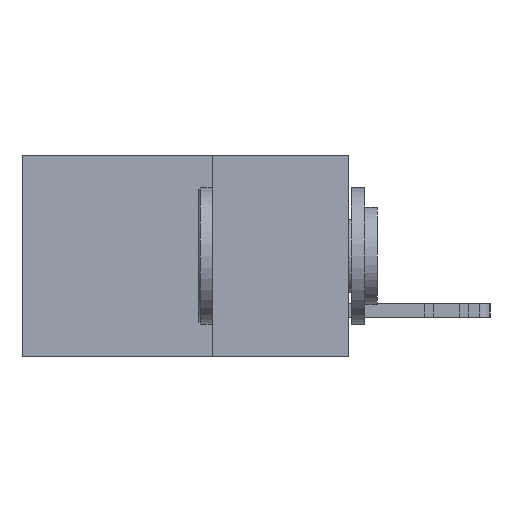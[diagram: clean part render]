
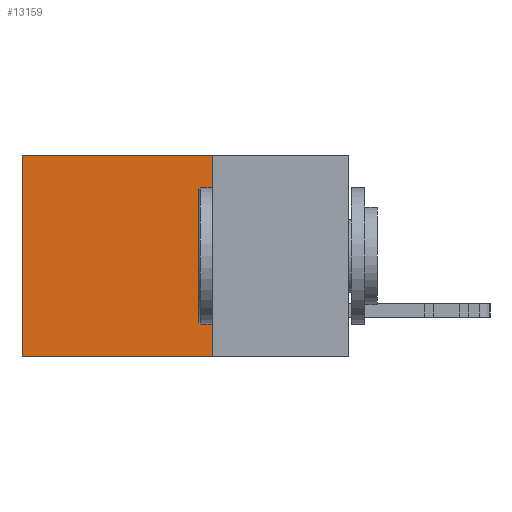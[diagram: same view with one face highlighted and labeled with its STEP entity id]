
A CAD part, left-side view. The second image highlights one B-rep face of the part: STEP entity #13159.
In plain terms, the highlighted planar face has unit normal (-1, 0, 0).
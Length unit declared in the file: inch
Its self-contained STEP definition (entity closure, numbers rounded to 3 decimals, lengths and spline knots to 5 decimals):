
#428 = EDGE_CURVE ( 'NONE', #21017, #10616, #10716, .T. ) ;
#1316 = DIRECTION ( 'NONE',  ( 1., 0., 0. ) ) ;
#2425 = VECTOR ( 'NONE', #23622, 39.37008 ) ;
#3263 = LINE ( 'NONE', #20273, #14201 ) ;
#3436 = LINE ( 'NONE', #19451, #26523 ) ;
#3722 = ORIENTED_EDGE ( 'NONE', *, *, #17890, .T. ) ;
#3991 = EDGE_CURVE ( 'NONE', #14884, #9442, #3263, .T. ) ;
#4906 = VECTOR ( 'NONE', #23539, 39.37008 ) ;
#6432 = DIRECTION ( 'NONE',  ( 0., 1., 0. ) ) ;
#7314 = CARTESIAN_POINT ( 'NONE',  ( 0.298, 0.25, 0. ) ) ;
#8314 = CARTESIAN_POINT ( 'NONE',  ( 0.298, 0.25, 0. ) ) ;
#9442 = VERTEX_POINT ( 'NONE', #20092 ) ;
#9477 = CARTESIAN_POINT ( 'NONE',  ( 0.298, 0.6, 0. ) ) ;
#10616 = VERTEX_POINT ( 'NONE', #16960 ) ;
#10716 = LINE ( 'NONE', #7314, #4906 ) ;
#12215 = CARTESIAN_POINT ( 'NONE',  ( 0.298, 0.25, 0. ) ) ;
#13159 = ADVANCED_FACE ( 'NONE', ( #27025 ), #23054, .F. ) ;
#14201 = VECTOR ( 'NONE', #17627, 39.37008 ) ;
#14769 = LINE ( 'NONE', #8314, #2425 ) ;
#14884 = VERTEX_POINT ( 'NONE', #9477 ) ;
#16430 = ORIENTED_EDGE ( 'NONE', *, *, #3991, .T. ) ;
#16613 = DIRECTION ( 'NONE',  ( 0., 0., -1. ) ) ;
#16960 = CARTESIAN_POINT ( 'NONE',  ( 0.298, 0.25, -0.37 ) ) ;
#17311 = EDGE_LOOP ( 'NONE', ( #16430, #21749, #17981, #3722 ) ) ;
#17627 = DIRECTION ( 'NONE',  ( 0., 0., -1. ) ) ;
#17890 = EDGE_CURVE ( 'NONE', #21017, #14884, #14769, .T. ) ;
#17981 = ORIENTED_EDGE ( 'NONE', *, *, #428, .F. ) ;
#19269 = CARTESIAN_POINT ( 'NONE',  ( 0.298, 0.25, 0. ) ) ;
#19451 = CARTESIAN_POINT ( 'NONE',  ( 0.298, 0.25, -0.37 ) ) ;
#20092 = CARTESIAN_POINT ( 'NONE',  ( 0.298, 0.6, -0.37 ) ) ;
#20273 = CARTESIAN_POINT ( 'NONE',  ( 0.298, 0.6, 0. ) ) ;
#21017 = VERTEX_POINT ( 'NONE', #19269 ) ;
#21072 = EDGE_CURVE ( 'NONE', #10616, #9442, #3436, .T. ) ;
#21749 = ORIENTED_EDGE ( 'NONE', *, *, #21072, .F. ) ;
#23054 = PLANE ( 'NONE',  #26004 ) ;
#23539 = DIRECTION ( 'NONE',  ( 0., 0., -1. ) ) ;
#23622 = DIRECTION ( 'NONE',  ( 0., 1., 0. ) ) ;
#26004 = AXIS2_PLACEMENT_3D ( 'NONE', #12215, #1316, #16613 ) ;
#26523 = VECTOR ( 'NONE', #6432, 39.37008 ) ;
#27025 = FACE_OUTER_BOUND ( 'NONE', #17311, .T. ) ;
